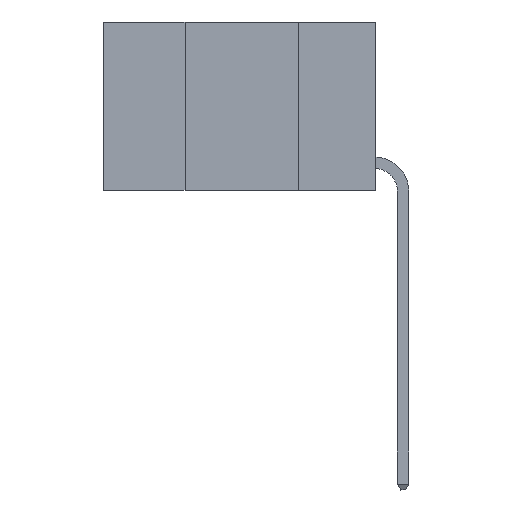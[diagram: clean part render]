
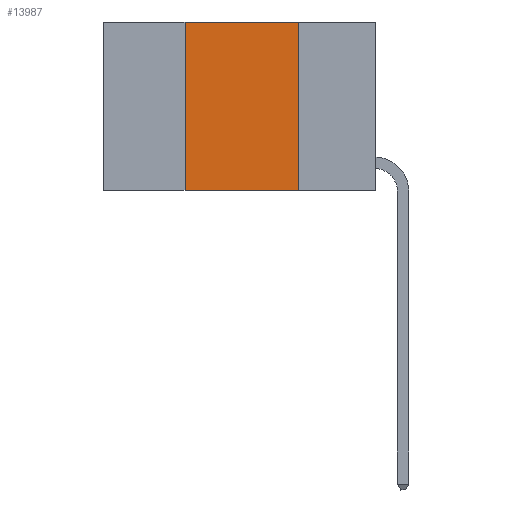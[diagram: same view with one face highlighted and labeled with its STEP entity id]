
A CAD part, left-side view. The second image highlights one B-rep face of the part: STEP entity #13987.
In plain terms, the highlighted planar face has unit normal (-1, 0, 0).
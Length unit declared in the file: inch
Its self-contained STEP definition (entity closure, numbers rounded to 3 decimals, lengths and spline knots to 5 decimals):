
#16 = DIRECTION ( 'NONE',  ( 0., -1., 0. ) ) ;
#127 = LINE ( 'NONE', #9672, #4399 ) ;
#446 = LINE ( 'NONE', #3404, #6351 ) ;
#557 = CARTESIAN_POINT ( 'NONE',  ( 0., 0.17, 0. ) ) ;
#1395 = LINE ( 'NONE', #1483, #2827 ) ;
#1483 = CARTESIAN_POINT ( 'NONE',  ( 0., 0.6, 0. ) ) ;
#1686 = DIRECTION ( 'NONE',  ( 0., 0., -1. ) ) ;
#2827 = VECTOR ( 'NONE', #4434, 39.37008 ) ;
#2907 = ORIENTED_EDGE ( 'NONE', *, *, #9952, .F. ) ;
#3404 = CARTESIAN_POINT ( 'NONE',  ( 0., 0.17, 0. ) ) ;
#4054 = FACE_OUTER_BOUND ( 'NONE', #14345, .T. ) ;
#4287 = CARTESIAN_POINT ( 'NONE',  ( 0., 0.17, -0.37 ) ) ;
#4309 = CARTESIAN_POINT ( 'NONE',  ( 0., 0.6, -0.37 ) ) ;
#4399 = VECTOR ( 'NONE', #16700, 39.37008 ) ;
#4434 = DIRECTION ( 'NONE',  ( 0., -1., 0. ) ) ;
#4444 = CARTESIAN_POINT ( 'NONE',  ( 0., 0.42, -0.37 ) ) ;
#6351 = VECTOR ( 'NONE', #1686, 39.37008 ) ;
#6620 = EDGE_CURVE ( 'NONE', #15555, #16438, #1395, .T. ) ;
#7520 = CARTESIAN_POINT ( 'NONE',  ( 0., 0.42, 0. ) ) ;
#9425 = VERTEX_POINT ( 'NONE', #4287 ) ;
#9672 = CARTESIAN_POINT ( 'NONE',  ( 0., 0.42, 0. ) ) ;
#9793 = CARTESIAN_POINT ( 'NONE',  ( 0., 0.6, 0. ) ) ;
#9810 = VERTEX_POINT ( 'NONE', #4444 ) ;
#9952 = EDGE_CURVE ( 'NONE', #16438, #9425, #446, .T. ) ;
#10534 = ORIENTED_EDGE ( 'NONE', *, *, #18358, .F. ) ;
#10692 = EDGE_CURVE ( 'NONE', #9810, #9425, #18890, .T. ) ;
#11328 = AXIS2_PLACEMENT_3D ( 'NONE', #9793, #13959, #16814 ) ;
#12522 = VECTOR ( 'NONE', #16, 39.37008 ) ;
#13959 = DIRECTION ( 'NONE',  ( 1., 0., 0. ) ) ;
#13987 = ADVANCED_FACE ( 'NONE', ( #4054 ), #15487, .F. ) ;
#14303 = ORIENTED_EDGE ( 'NONE', *, *, #6620, .F. ) ;
#14345 = EDGE_LOOP ( 'NONE', ( #2907, #14303, #10534, #18584 ) ) ;
#15487 = PLANE ( 'NONE',  #11328 ) ;
#15555 = VERTEX_POINT ( 'NONE', #7520 ) ;
#16438 = VERTEX_POINT ( 'NONE', #557 ) ;
#16700 = DIRECTION ( 'NONE',  ( 0., 0., 1. ) ) ;
#16814 = DIRECTION ( 'NONE',  ( 0., 0., -1. ) ) ;
#18358 = EDGE_CURVE ( 'NONE', #9810, #15555, #127, .T. ) ;
#18584 = ORIENTED_EDGE ( 'NONE', *, *, #10692, .T. ) ;
#18890 = LINE ( 'NONE', #4309, #12522 ) ;
